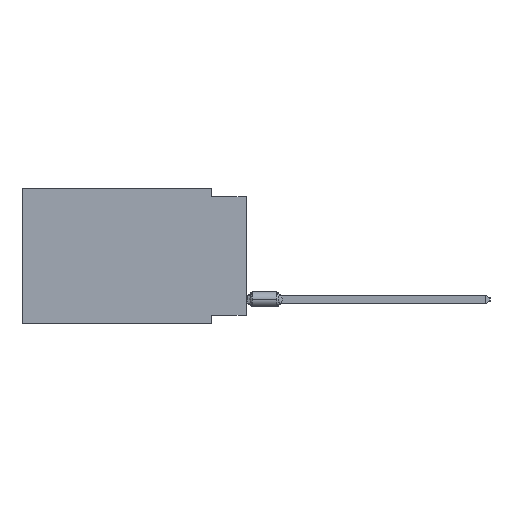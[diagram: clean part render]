
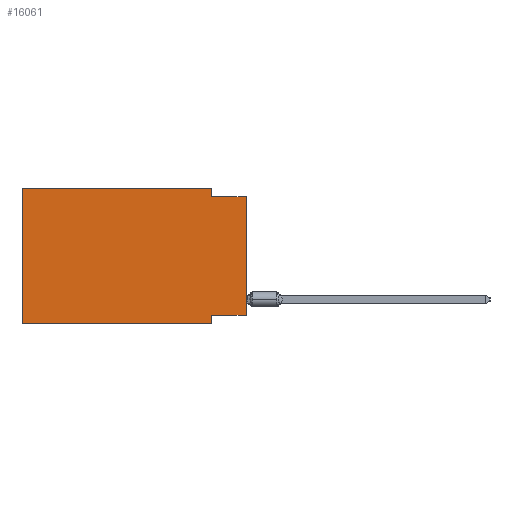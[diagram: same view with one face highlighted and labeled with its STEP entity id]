
A CAD part, left-side view. The second image highlights one B-rep face of the part: STEP entity #16061.
In plain terms, the highlighted planar face has unit normal (-1, 0, 0).
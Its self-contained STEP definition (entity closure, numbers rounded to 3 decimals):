
#572 = DIRECTION ( 'NONE',  ( 0., 0., 1. ) ) ;
#3421 = CARTESIAN_POINT ( 'NONE',  ( 0., 2.54, 0. ) ) ;
#3480 = DIRECTION ( 'NONE',  ( 1., 0., 0. ) ) ;
#4563 = EDGE_CURVE ( 'NONE', #19189, #25842, #14063, .T. ) ;
#6193 = CARTESIAN_POINT ( 'NONE',  ( 0., 2.54, 0. ) ) ;
#6582 = CARTESIAN_POINT ( 'NONE',  ( 0., 0., -9.271 ) ) ;
#7443 = VECTOR ( 'NONE', #36348, 1000. ) ;
#8275 = CARTESIAN_POINT ( 'NONE',  ( 0., 16.383, 0. ) ) ;
#8440 = LINE ( 'NONE', #22826, #7443 ) ;
#9309 = EDGE_CURVE ( 'NONE', #40949, #19189, #48440, .T. ) ;
#10365 = VECTOR ( 'NONE', #18399, 1000. ) ;
#12606 = ORIENTED_EDGE ( 'NONE', *, *, #20475, .F. ) ;
#13055 = CARTESIAN_POINT ( 'NONE',  ( 0., 2.54, -9.906 ) ) ;
#14063 = LINE ( 'NONE', #27866, #45189 ) ;
#14119 = VECTOR ( 'NONE', #31794, 1000. ) ;
#14380 = VERTEX_POINT ( 'NONE', #42750 ) ;
#15235 = ORIENTED_EDGE ( 'NONE', *, *, #30140, .T. ) ;
#16061 = ADVANCED_FACE ( 'NONE', ( #21476 ), #40106, .F. ) ;
#18399 = DIRECTION ( 'NONE',  ( 0., 0., 1. ) ) ;
#18590 = LINE ( 'NONE', #50414, #14119 ) ;
#19189 = VERTEX_POINT ( 'NONE', #58931 ) ;
#20475 = EDGE_CURVE ( 'NONE', #52416, #23432, #18590, .T. ) ;
#20571 = VECTOR ( 'NONE', #24880, 1000. ) ;
#21415 = DIRECTION ( 'NONE',  ( 0., -1., 0. ) ) ;
#21476 = FACE_OUTER_BOUND ( 'NONE', #34385, .T. ) ;
#22826 = CARTESIAN_POINT ( 'NONE',  ( 0., 16.383, 0. ) ) ;
#23432 = VERTEX_POINT ( 'NONE', #13055 ) ;
#23657 = LINE ( 'NONE', #41981, #57341 ) ;
#24160 = VERTEX_POINT ( 'NONE', #31328 ) ;
#24880 = DIRECTION ( 'NONE',  ( 0., 1., 0. ) ) ;
#25189 = EDGE_CURVE ( 'NONE', #14380, #52416, #51917, .T. ) ;
#25842 = VERTEX_POINT ( 'NONE', #39676 ) ;
#26911 = ORIENTED_EDGE ( 'NONE', *, *, #58970, .F. ) ;
#27866 = CARTESIAN_POINT ( 'NONE',  ( 0., 0., -0.635 ) ) ;
#27916 = ORIENTED_EDGE ( 'NONE', *, *, #30544, .F. ) ;
#30140 = EDGE_CURVE ( 'NONE', #14380, #25842, #31606, .T. ) ;
#30404 = CARTESIAN_POINT ( 'NONE',  ( 0., 16.383, -9.906 ) ) ;
#30544 = EDGE_CURVE ( 'NONE', #38245, #40949, #8440, .T. ) ;
#31278 = ORIENTED_EDGE ( 'NONE', *, *, #25189, .F. ) ;
#31328 = CARTESIAN_POINT ( 'NONE',  ( 0., 16.383, -9.906 ) ) ;
#31606 = LINE ( 'NONE', #55651, #10365 ) ;
#31794 = DIRECTION ( 'NONE',  ( 0., 0., -1. ) ) ;
#34385 = EDGE_LOOP ( 'NONE', ( #15235, #39267, #53990, #27916, #26911, #54339, #12606, #31278 ) ) ;
#36348 = DIRECTION ( 'NONE',  ( 0., -1., 0. ) ) ;
#36635 = LINE ( 'NONE', #30404, #58289 ) ;
#38245 = VERTEX_POINT ( 'NONE', #45721 ) ;
#39267 = ORIENTED_EDGE ( 'NONE', *, *, #4563, .F. ) ;
#39676 = CARTESIAN_POINT ( 'NONE',  ( 0., 0., -0.635 ) ) ;
#40106 = PLANE ( 'NONE',  #44239 ) ;
#40949 = VERTEX_POINT ( 'NONE', #6193 ) ;
#41981 = CARTESIAN_POINT ( 'NONE',  ( 0., 16.383, 0. ) ) ;
#42750 = CARTESIAN_POINT ( 'NONE',  ( 0., 0., -9.271 ) ) ;
#44239 = AXIS2_PLACEMENT_3D ( 'NONE', #8275, #3480, #48819 ) ;
#45189 = VECTOR ( 'NONE', #46190, 1000. ) ;
#45721 = CARTESIAN_POINT ( 'NONE',  ( 0., 16.383, 0. ) ) ;
#46190 = DIRECTION ( 'NONE',  ( 0., -1., 0. ) ) ;
#46440 = CARTESIAN_POINT ( 'NONE',  ( 0., 2.54, -9.271 ) ) ;
#48440 = LINE ( 'NONE', #3421, #51335 ) ;
#48819 = DIRECTION ( 'NONE',  ( 0., 0., -1. ) ) ;
#49052 = DIRECTION ( 'NONE',  ( 0., 0., -1. ) ) ;
#50414 = CARTESIAN_POINT ( 'NONE',  ( 0., 2.54, -9.906 ) ) ;
#51335 = VECTOR ( 'NONE', #49052, 1000. ) ;
#51917 = LINE ( 'NONE', #6582, #20571 ) ;
#52416 = VERTEX_POINT ( 'NONE', #46440 ) ;
#53990 = ORIENTED_EDGE ( 'NONE', *, *, #9309, .F. ) ;
#54339 = ORIENTED_EDGE ( 'NONE', *, *, #58445, .T. ) ;
#55651 = CARTESIAN_POINT ( 'NONE',  ( 0., 0., 0. ) ) ;
#57341 = VECTOR ( 'NONE', #572, 1000. ) ;
#58289 = VECTOR ( 'NONE', #21415, 1000. ) ;
#58445 = EDGE_CURVE ( 'NONE', #24160, #23432, #36635, .T. ) ;
#58931 = CARTESIAN_POINT ( 'NONE',  ( 0., 2.54, -0.635 ) ) ;
#58970 = EDGE_CURVE ( 'NONE', #24160, #38245, #23657, .T. ) ;
